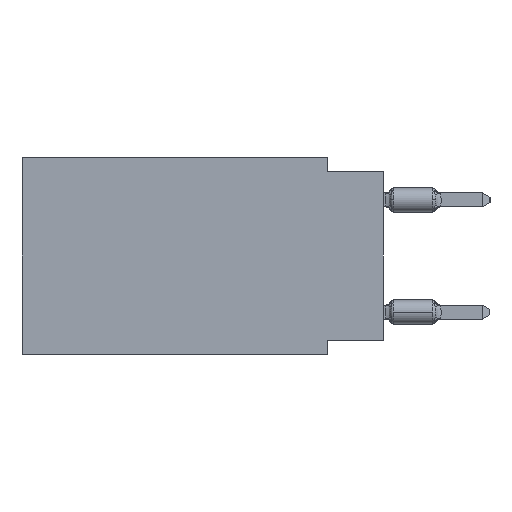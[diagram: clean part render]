
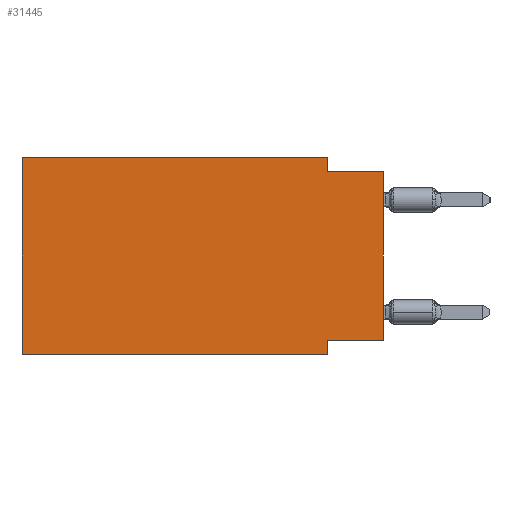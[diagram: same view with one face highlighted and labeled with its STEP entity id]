
A CAD part, left-side view. The second image highlights one B-rep face of the part: STEP entity #31445.
In plain terms, the highlighted planar face has unit normal (-1, 0, 0).
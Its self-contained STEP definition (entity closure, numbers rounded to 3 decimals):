
#71 = ORIENTED_EDGE ( 'NONE', *, *, #10173, .T. ) ;
#1280 = CARTESIAN_POINT ( 'NONE',  ( 0., 16.383, 0. ) ) ;
#1639 = CARTESIAN_POINT ( 'NONE',  ( 0., 0., 0. ) ) ;
#2413 = EDGE_CURVE ( 'NONE', #7970, #8045, #25826, .T. ) ;
#3328 = EDGE_CURVE ( 'NONE', #35544, #36296, #30293, .T. ) ;
#3614 = ORIENTED_EDGE ( 'NONE', *, *, #32671, .F. ) ;
#3855 = CARTESIAN_POINT ( 'NONE',  ( 0., 2.54, -8.89 ) ) ;
#4347 = EDGE_CURVE ( 'NONE', #36296, #7970, #15245, .T. ) ;
#6137 = VECTOR ( 'NONE', #20030, 1000. ) ;
#6441 = VERTEX_POINT ( 'NONE', #20758 ) ;
#7472 = CARTESIAN_POINT ( 'NONE',  ( 0., 2.54, -8.255 ) ) ;
#7707 = VECTOR ( 'NONE', #35676, 1000. ) ;
#7970 = VERTEX_POINT ( 'NONE', #9363 ) ;
#8045 = VERTEX_POINT ( 'NONE', #16769 ) ;
#9363 = CARTESIAN_POINT ( 'NONE',  ( 0., 2.54, 0. ) ) ;
#9426 = CARTESIAN_POINT ( 'NONE',  ( 0., 0., -8.255 ) ) ;
#9917 = LINE ( 'NONE', #16474, #41304 ) ;
#10173 = EDGE_CURVE ( 'NONE', #6441, #19825, #18225, .T. ) ;
#11321 = LINE ( 'NONE', #18727, #42373 ) ;
#12478 = EDGE_CURVE ( 'NONE', #35544, #29823, #11321, .T. ) ;
#12495 = DIRECTION ( 'NONE',  ( 0., 0., -1. ) ) ;
#12776 = DIRECTION ( 'NONE',  ( 0., -1., 0. ) ) ;
#13891 = CARTESIAN_POINT ( 'NONE',  ( 0., 16.383, 0. ) ) ;
#13922 = ORIENTED_EDGE ( 'NONE', *, *, #3328, .F. ) ;
#14713 = DIRECTION ( 'NONE',  ( 0., 0., -1. ) ) ;
#15137 = CARTESIAN_POINT ( 'NONE',  ( 0., 16.383, 0. ) ) ;
#15245 = LINE ( 'NONE', #1280, #17390 ) ;
#16474 = CARTESIAN_POINT ( 'NONE',  ( 0., 0., -0.635 ) ) ;
#16769 = CARTESIAN_POINT ( 'NONE',  ( 0., 2.54, -0.635 ) ) ;
#17390 = VECTOR ( 'NONE', #41684, 1000. ) ;
#18015 = EDGE_LOOP ( 'NONE', ( #71, #39472, #24387, #31056, #13922, #33214, #3614, #41324 ) ) ;
#18020 = VERTEX_POINT ( 'NONE', #7472 ) ;
#18225 = LINE ( 'NONE', #1639, #7707 ) ;
#18727 = CARTESIAN_POINT ( 'NONE',  ( 0., 16.383, -8.89 ) ) ;
#19825 = VERTEX_POINT ( 'NONE', #42792 ) ;
#20023 = VECTOR ( 'NONE', #35863, 1000. ) ;
#20030 = DIRECTION ( 'NONE',  ( 0., 0., 1. ) ) ;
#20758 = CARTESIAN_POINT ( 'NONE',  ( 0., 0., -8.255 ) ) ;
#22560 = CARTESIAN_POINT ( 'NONE',  ( 0., 2.54, 0. ) ) ;
#23406 = DIRECTION ( 'NONE',  ( 0., 1., 0. ) ) ;
#23826 = VECTOR ( 'NONE', #23406, 1000. ) ;
#23906 = FACE_OUTER_BOUND ( 'NONE', #18015, .T. ) ;
#24387 = ORIENTED_EDGE ( 'NONE', *, *, #2413, .F. ) ;
#25759 = AXIS2_PLACEMENT_3D ( 'NONE', #15137, #38721, #12495 ) ;
#25826 = LINE ( 'NONE', #22560, #20023 ) ;
#27398 = LINE ( 'NONE', #31301, #37696 ) ;
#27799 = EDGE_CURVE ( 'NONE', #8045, #19825, #9917, .T. ) ;
#29792 = CARTESIAN_POINT ( 'NONE',  ( 0., 16.383, -8.89 ) ) ;
#29823 = VERTEX_POINT ( 'NONE', #3855 ) ;
#30293 = LINE ( 'NONE', #13891, #6137 ) ;
#31056 = ORIENTED_EDGE ( 'NONE', *, *, #4347, .F. ) ;
#31301 = CARTESIAN_POINT ( 'NONE',  ( 0., 2.54, -8.89 ) ) ;
#31445 = ADVANCED_FACE ( 'NONE', ( #23906 ), #37222, .F. ) ;
#32039 = DIRECTION ( 'NONE',  ( 0., -1., 0. ) ) ;
#32671 = EDGE_CURVE ( 'NONE', #18020, #29823, #27398, .T. ) ;
#33214 = ORIENTED_EDGE ( 'NONE', *, *, #12478, .T. ) ;
#35363 = CARTESIAN_POINT ( 'NONE',  ( 0., 16.383, 0. ) ) ;
#35544 = VERTEX_POINT ( 'NONE', #29792 ) ;
#35676 = DIRECTION ( 'NONE',  ( 0., 0., 1. ) ) ;
#35863 = DIRECTION ( 'NONE',  ( 0., 0., -1. ) ) ;
#35931 = EDGE_CURVE ( 'NONE', #6441, #18020, #39344, .T. ) ;
#36296 = VERTEX_POINT ( 'NONE', #35363 ) ;
#37222 = PLANE ( 'NONE',  #25759 ) ;
#37696 = VECTOR ( 'NONE', #14713, 1000. ) ;
#38721 = DIRECTION ( 'NONE',  ( 1., 0., 0. ) ) ;
#39344 = LINE ( 'NONE', #9426, #23826 ) ;
#39472 = ORIENTED_EDGE ( 'NONE', *, *, #27799, .F. ) ;
#41304 = VECTOR ( 'NONE', #12776, 1000. ) ;
#41324 = ORIENTED_EDGE ( 'NONE', *, *, #35931, .F. ) ;
#41684 = DIRECTION ( 'NONE',  ( 0., -1., 0. ) ) ;
#42373 = VECTOR ( 'NONE', #32039, 1000. ) ;
#42792 = CARTESIAN_POINT ( 'NONE',  ( 0., 0., -0.635 ) ) ;
